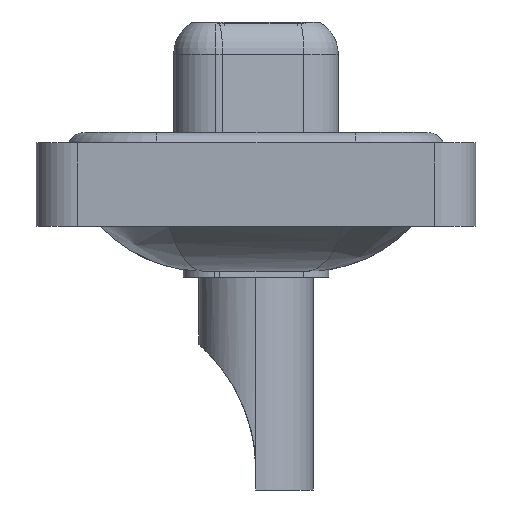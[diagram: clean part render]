
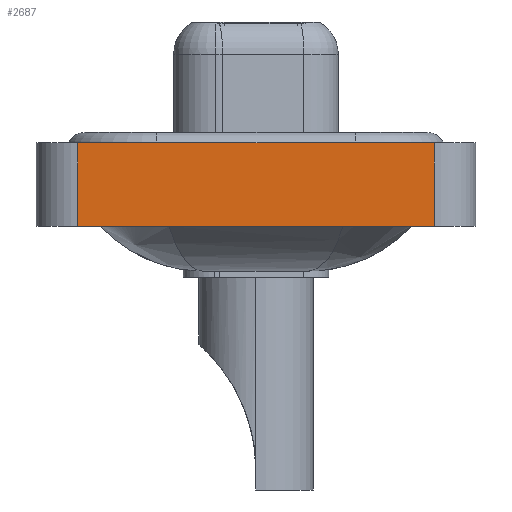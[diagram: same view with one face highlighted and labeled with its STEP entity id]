
A CAD part, left-side view. The second image highlights one B-rep face of the part: STEP entity #2687.
In plain terms, the highlighted planar face has unit normal (-1, 0, 0).
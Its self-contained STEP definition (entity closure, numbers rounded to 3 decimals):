
#393 = DIRECTION ( 'NONE',  ( 0., 0., 1. ) ) ;
#1194 = VECTOR ( 'NONE', #393, 1000. ) ;
#1670 = FACE_OUTER_BOUND ( 'NONE', #14904, .T. ) ;
#1756 = PLANE ( 'NONE',  #2497 ) ;
#2043 = CARTESIAN_POINT ( 'NONE',  ( -7.3, -8.55, -3.6 ) ) ;
#2459 = CARTESIAN_POINT ( 'NONE',  ( -7.3, -8.55, 0.4 ) ) ;
#2497 = AXIS2_PLACEMENT_3D ( 'NONE', #2990, #11540, #14406 ) ;
#2687 = ADVANCED_FACE ( 'NONE', ( #1670 ), #1756, .T. ) ;
#2865 = ORIENTED_EDGE ( 'NONE', *, *, #13268, .F. ) ;
#2990 = CARTESIAN_POINT ( 'NONE',  ( -7.3, -8.55, -3.6 ) ) ;
#3059 = LINE ( 'NONE', #8045, #11454 ) ;
#3175 = VECTOR ( 'NONE', #4111, 1000. ) ;
#3195 = LINE ( 'NONE', #15602, #3175 ) ;
#3686 = VERTEX_POINT ( 'NONE', #2459 ) ;
#3915 = CARTESIAN_POINT ( 'NONE',  ( -7.3, -8.55, -3.6 ) ) ;
#4111 = DIRECTION ( 'NONE',  ( 0., -1., 0. ) ) ;
#5064 = ORIENTED_EDGE ( 'NONE', *, *, #7030, .T. ) ;
#5317 = DIRECTION ( 'NONE',  ( 0., 0., 1. ) ) ;
#5922 = CARTESIAN_POINT ( 'NONE',  ( -7.3, 8.55, 0.4 ) ) ;
#6608 = CARTESIAN_POINT ( 'NONE',  ( -7.3, -8.55, -3.6 ) ) ;
#7030 = EDGE_CURVE ( 'NONE', #12368, #8046, #9980, .T. ) ;
#8045 = CARTESIAN_POINT ( 'NONE',  ( -7.3, 8.55, -3.6 ) ) ;
#8046 = VERTEX_POINT ( 'NONE', #2043 ) ;
#8101 = ORIENTED_EDGE ( 'NONE', *, *, #14519, .F. ) ;
#9980 = LINE ( 'NONE', #3915, #10342 ) ;
#10342 = VECTOR ( 'NONE', #11301, 1000. ) ;
#10456 = CARTESIAN_POINT ( 'NONE',  ( -7.3, 8.55, -3.6 ) ) ;
#10981 = ORIENTED_EDGE ( 'NONE', *, *, #15572, .T. ) ;
#11301 = DIRECTION ( 'NONE',  ( 0., -1., 0. ) ) ;
#11454 = VECTOR ( 'NONE', #5317, 1000. ) ;
#11540 = DIRECTION ( 'NONE',  ( -1., 0., 0. ) ) ;
#11738 = LINE ( 'NONE', #6608, #1194 ) ;
#11767 = VERTEX_POINT ( 'NONE', #5922 ) ;
#12368 = VERTEX_POINT ( 'NONE', #10456 ) ;
#13268 = EDGE_CURVE ( 'NONE', #11767, #3686, #3195, .T. ) ;
#14406 = DIRECTION ( 'NONE',  ( 0., 0., 1. ) ) ;
#14519 = EDGE_CURVE ( 'NONE', #12368, #11767, #3059, .T. ) ;
#14904 = EDGE_LOOP ( 'NONE', ( #10981, #2865, #8101, #5064 ) ) ;
#15572 = EDGE_CURVE ( 'NONE', #8046, #3686, #11738, .T. ) ;
#15602 = CARTESIAN_POINT ( 'NONE',  ( -7.3, -8.55, 0.4 ) ) ;
